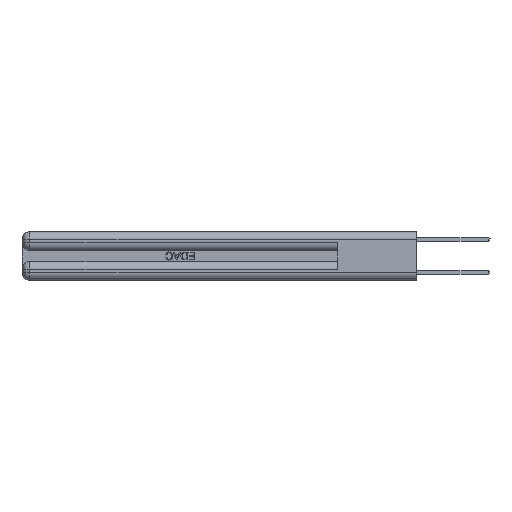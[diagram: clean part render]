
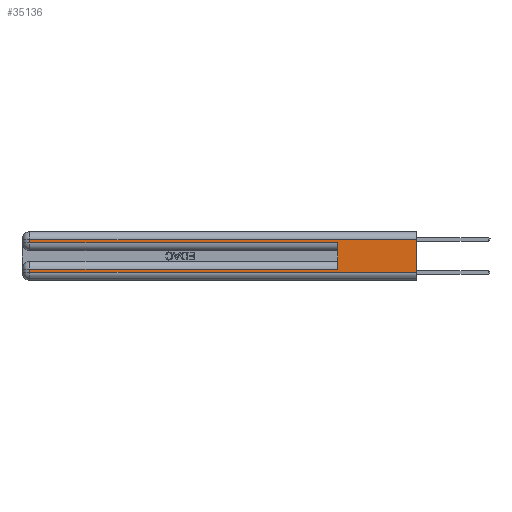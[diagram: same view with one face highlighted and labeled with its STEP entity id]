
A CAD part, left-side view. The second image highlights one B-rep face of the part: STEP entity #35136.
In plain terms, the highlighted planar face has unit normal (-1, 0, 0).
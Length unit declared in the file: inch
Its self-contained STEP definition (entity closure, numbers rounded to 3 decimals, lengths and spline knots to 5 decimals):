
#260 = LINE ( 'NONE', #30177, #13867 ) ;
#317 = VECTOR ( 'NONE', #2561, 39.37008 ) ;
#1648 = ORIENTED_EDGE ( 'NONE', *, *, #16300, .T. ) ;
#1815 = DIRECTION ( 'NONE',  ( 0., -1., 0. ) ) ;
#2212 = FACE_OUTER_BOUND ( 'NONE', #25069, .T. ) ;
#2321 = CARTESIAN_POINT ( 'NONE',  ( 0., 2.94, 0.285 ) ) ;
#2450 = PLANE ( 'NONE',  #15798 ) ;
#2561 = DIRECTION ( 'NONE',  ( 0., 1., 0. ) ) ;
#3355 = CARTESIAN_POINT ( 'NONE',  ( 0., 2.94, 0.37 ) ) ;
#3915 = LINE ( 'NONE', #29402, #8958 ) ;
#4225 = VERTEX_POINT ( 'NONE', #27371 ) ;
#4750 = ORIENTED_EDGE ( 'NONE', *, *, #27339, .T. ) ;
#5457 = VECTOR ( 'NONE', #27892, 39.37008 ) ;
#7335 = LINE ( 'NONE', #9909, #14191 ) ;
#7693 = EDGE_CURVE ( 'NONE', #29883, #12219, #30534, .T. ) ;
#8081 = ORIENTED_EDGE ( 'NONE', *, *, #13779, .T. ) ;
#8716 = VECTOR ( 'NONE', #29560, 39.37008 ) ;
#8958 = VECTOR ( 'NONE', #10447, 39.37008 ) ;
#9253 = EDGE_CURVE ( 'NONE', #29883, #20696, #260, .T. ) ;
#9670 = ORIENTED_EDGE ( 'NONE', *, *, #19268, .T. ) ;
#9762 = EDGE_CURVE ( 'NONE', #29235, #21461, #26774, .T. ) ;
#9909 = CARTESIAN_POINT ( 'NONE',  ( 0., 0., 0.06 ) ) ;
#10447 = DIRECTION ( 'NONE',  ( 0., 0., 1. ) ) ;
#10531 = DIRECTION ( 'NONE',  ( 1., 0., 0. ) ) ;
#10656 = DIRECTION ( 'NONE',  ( 0., 0., -1. ) ) ;
#10736 = CARTESIAN_POINT ( 'NONE',  ( 0., 2.94, 0.37 ) ) ;
#12161 = EDGE_CURVE ( 'NONE', #22079, #21461, #3915, .T. ) ;
#12219 = VERTEX_POINT ( 'NONE', #13546 ) ;
#12766 = VERTEX_POINT ( 'NONE', #30612 ) ;
#13546 = CARTESIAN_POINT ( 'NONE',  ( 0., 0., 0.06 ) ) ;
#13779 = EDGE_CURVE ( 'NONE', #20696, #29235, #24683, .T. ) ;
#13867 = VECTOR ( 'NONE', #33252, 39.37008 ) ;
#14191 = VECTOR ( 'NONE', #15389, 39.37008 ) ;
#14371 = CARTESIAN_POINT ( 'NONE',  ( 0., 0.6, 0.085 ) ) ;
#14786 = LINE ( 'NONE', #29694, #317 ) ;
#15366 = CARTESIAN_POINT ( 'NONE',  ( 0., 0., 0.285 ) ) ;
#15389 = DIRECTION ( 'NONE',  ( 0., -1., 0. ) ) ;
#15798 = AXIS2_PLACEMENT_3D ( 'NONE', #35183, #10531, #10656 ) ;
#16012 = LINE ( 'NONE', #10736, #8716 ) ;
#16203 = CARTESIAN_POINT ( 'NONE',  ( 0., 0., 0.31 ) ) ;
#16300 = EDGE_CURVE ( 'NONE', #4225, #12766, #16012, .T. ) ;
#18189 = ORIENTED_EDGE ( 'NONE', *, *, #7693, .F. ) ;
#19268 = EDGE_CURVE ( 'NONE', #12766, #12219, #7335, .T. ) ;
#20384 = VECTOR ( 'NONE', #1815, 39.37008 ) ;
#20696 = VERTEX_POINT ( 'NONE', #34810 ) ;
#21461 = VERTEX_POINT ( 'NONE', #25868 ) ;
#21545 = CARTESIAN_POINT ( 'NONE',  ( 0., 0., 0.37 ) ) ;
#22079 = VERTEX_POINT ( 'NONE', #14371 ) ;
#24008 = ORIENTED_EDGE ( 'NONE', *, *, #12161, .F. ) ;
#24683 = LINE ( 'NONE', #3355, #5457 ) ;
#25069 = EDGE_LOOP ( 'NONE', ( #18189, #31151, #8081, #26400, #24008, #4750, #1648, #9670 ) ) ;
#25868 = CARTESIAN_POINT ( 'NONE',  ( 0., 0.6, 0.285 ) ) ;
#26400 = ORIENTED_EDGE ( 'NONE', *, *, #9762, .T. ) ;
#26672 = DIRECTION ( 'NONE',  ( 0., 0., -1. ) ) ;
#26774 = LINE ( 'NONE', #15366, #20384 ) ;
#27339 = EDGE_CURVE ( 'NONE', #22079, #4225, #14786, .T. ) ;
#27371 = CARTESIAN_POINT ( 'NONE',  ( 0., 2.94, 0.085 ) ) ;
#27892 = DIRECTION ( 'NONE',  ( 0., 0., -1. ) ) ;
#29235 = VERTEX_POINT ( 'NONE', #2321 ) ;
#29402 = CARTESIAN_POINT ( 'NONE',  ( 0., 0.6, 0.145 ) ) ;
#29560 = DIRECTION ( 'NONE',  ( 0., 0., -1. ) ) ;
#29694 = CARTESIAN_POINT ( 'NONE',  ( 0., 0., 0.085 ) ) ;
#29748 = VECTOR ( 'NONE', #26672, 39.37008 ) ;
#29883 = VERTEX_POINT ( 'NONE', #16203 ) ;
#30177 = CARTESIAN_POINT ( 'NONE',  ( 0., 0., 0.31 ) ) ;
#30534 = LINE ( 'NONE', #21545, #29748 ) ;
#30612 = CARTESIAN_POINT ( 'NONE',  ( 0., 2.94, 0.06 ) ) ;
#31151 = ORIENTED_EDGE ( 'NONE', *, *, #9253, .T. ) ;
#33252 = DIRECTION ( 'NONE',  ( 0., 1., 0. ) ) ;
#34810 = CARTESIAN_POINT ( 'NONE',  ( 0., 2.94, 0.31 ) ) ;
#35136 = ADVANCED_FACE ( 'NONE', ( #2212 ), #2450, .F. ) ;
#35183 = CARTESIAN_POINT ( 'NONE',  ( 0., 0., 0.37 ) ) ;
